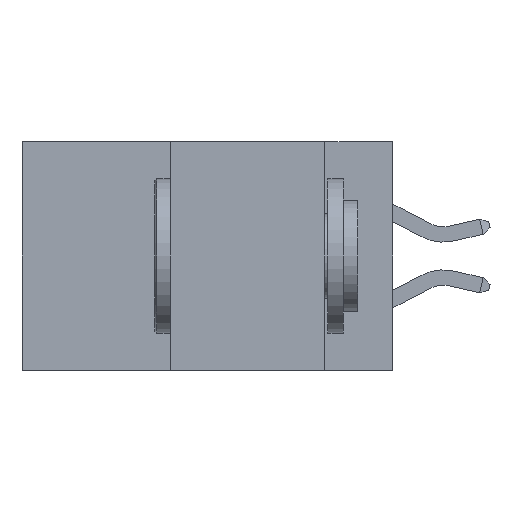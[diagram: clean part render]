
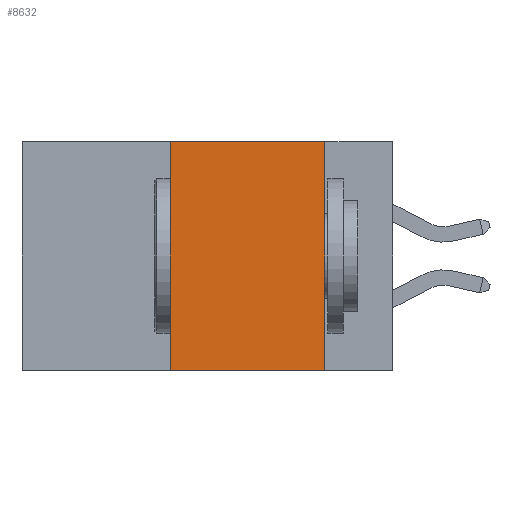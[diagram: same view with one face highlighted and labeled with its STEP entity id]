
A CAD part, left-side view. The second image highlights one B-rep face of the part: STEP entity #8632.
In plain terms, the highlighted planar face has unit normal (-1, 0, 0).
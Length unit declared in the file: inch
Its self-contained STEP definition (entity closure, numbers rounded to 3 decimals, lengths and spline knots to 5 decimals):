
#779 = ORIENTED_EDGE ( 'NONE', *, *, #7772, .F. ) ;
#964 = CARTESIAN_POINT ( 'NONE',  ( 0., 0.11, -0.37 ) ) ;
#1034 = VECTOR ( 'NONE', #2395, 39.37008 ) ;
#1516 = EDGE_LOOP ( 'NONE', ( #779, #2787, #3158, #8747 ) ) ;
#1764 = CARTESIAN_POINT ( 'NONE',  ( 0., 0.36, 0. ) ) ;
#2116 = VERTEX_POINT ( 'NONE', #1764 ) ;
#2395 = DIRECTION ( 'NONE',  ( 0., 0., -1. ) ) ;
#2787 = ORIENTED_EDGE ( 'NONE', *, *, #12139, .F. ) ;
#3158 = ORIENTED_EDGE ( 'NONE', *, *, #3974, .F. ) ;
#3338 = LINE ( 'NONE', #5955, #9058 ) ;
#3381 = CARTESIAN_POINT ( 'NONE',  ( 0., 0.11, 0. ) ) ;
#3956 = LINE ( 'NONE', #9614, #11832 ) ;
#3974 = EDGE_CURVE ( 'NONE', #10811, #2116, #3956, .T. ) ;
#4176 = VERTEX_POINT ( 'NONE', #6297 ) ;
#4408 = VECTOR ( 'NONE', #7373, 39.37008 ) ;
#4870 = EDGE_CURVE ( 'NONE', #10811, #7014, #3338, .T. ) ;
#5955 = CARTESIAN_POINT ( 'NONE',  ( 0., 0.6, -0.37 ) ) ;
#6249 = CARTESIAN_POINT ( 'NONE',  ( 0., 0.6, 0. ) ) ;
#6297 = CARTESIAN_POINT ( 'NONE',  ( 0., 0.11, 0. ) ) ;
#6321 = CARTESIAN_POINT ( 'NONE',  ( 0., 0.6, 0. ) ) ;
#6517 = CARTESIAN_POINT ( 'NONE',  ( 0., 0.36, -0.37 ) ) ;
#7014 = VERTEX_POINT ( 'NONE', #964 ) ;
#7373 = DIRECTION ( 'NONE',  ( 0., -1., 0. ) ) ;
#7772 = EDGE_CURVE ( 'NONE', #4176, #7014, #11895, .T. ) ;
#8512 = DIRECTION ( 'NONE',  ( 0., 0., -1. ) ) ;
#8632 = ADVANCED_FACE ( 'NONE', ( #9720 ), #9223, .F. ) ;
#8747 = ORIENTED_EDGE ( 'NONE', *, *, #4870, .T. ) ;
#9058 = VECTOR ( 'NONE', #11786, 39.37008 ) ;
#9223 = PLANE ( 'NONE',  #11775 ) ;
#9316 = DIRECTION ( 'NONE',  ( 1., 0., 0. ) ) ;
#9614 = CARTESIAN_POINT ( 'NONE',  ( 0., 0.36, 0. ) ) ;
#9720 = FACE_OUTER_BOUND ( 'NONE', #1516, .T. ) ;
#10811 = VERTEX_POINT ( 'NONE', #6517 ) ;
#10917 = DIRECTION ( 'NONE',  ( 0., 0., 1. ) ) ;
#11543 = LINE ( 'NONE', #6321, #4408 ) ;
#11775 = AXIS2_PLACEMENT_3D ( 'NONE', #6249, #9316, #8512 ) ;
#11786 = DIRECTION ( 'NONE',  ( 0., -1., 0. ) ) ;
#11832 = VECTOR ( 'NONE', #10917, 39.37008 ) ;
#11895 = LINE ( 'NONE', #3381, #1034 ) ;
#12139 = EDGE_CURVE ( 'NONE', #2116, #4176, #11543, .T. ) ;
